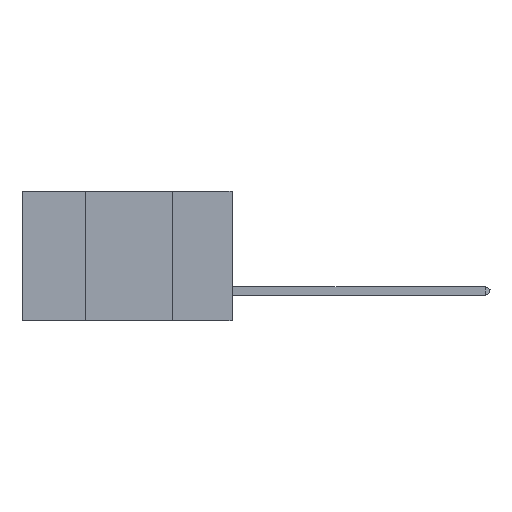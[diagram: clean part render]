
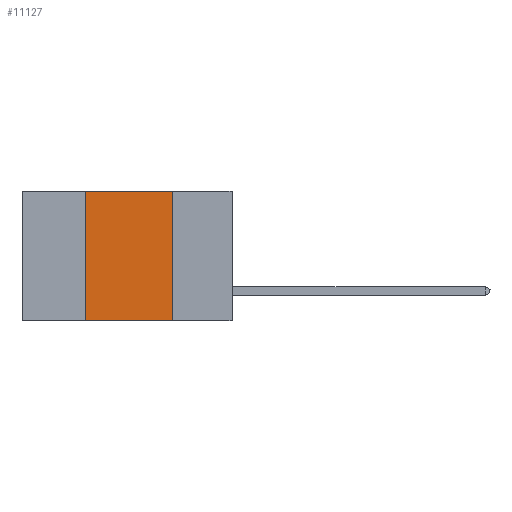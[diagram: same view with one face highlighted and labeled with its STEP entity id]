
A CAD part, left-side view. The second image highlights one B-rep face of the part: STEP entity #11127.
In plain terms, the highlighted planar face has unit normal (-1, 0, 0).
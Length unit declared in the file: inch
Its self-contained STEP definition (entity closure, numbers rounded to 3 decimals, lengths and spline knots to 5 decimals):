
#441 = ORIENTED_EDGE ( 'NONE', *, *, #6847, .F. ) ;
#1531 = CARTESIAN_POINT ( 'NONE',  ( 0., 0.42, -0.37 ) ) ;
#1762 = VERTEX_POINT ( 'NONE', #1531 ) ;
#2205 = LINE ( 'NONE', #15327, #3920 ) ;
#2285 = EDGE_CURVE ( 'NONE', #1762, #3247, #2205, .T. ) ;
#2792 = PLANE ( 'NONE',  #5983 ) ;
#3013 = CARTESIAN_POINT ( 'NONE',  ( 0., 0.6, 0. ) ) ;
#3247 = VERTEX_POINT ( 'NONE', #8377 ) ;
#3689 = LINE ( 'NONE', #3013, #16698 ) ;
#3920 = VECTOR ( 'NONE', #15156, 39.37008 ) ;
#4222 = DIRECTION ( 'NONE',  ( 1., 0., 0. ) ) ;
#4903 = CARTESIAN_POINT ( 'NONE',  ( 0., 0.17, 0. ) ) ;
#5390 = VERTEX_POINT ( 'NONE', #16232 ) ;
#5679 = CARTESIAN_POINT ( 'NONE',  ( 0., 0.42, 0. ) ) ;
#5760 = EDGE_CURVE ( 'NONE', #1762, #11812, #14618, .T. ) ;
#5983 = AXIS2_PLACEMENT_3D ( 'NONE', #8307, #4222, #11189 ) ;
#6644 = ORIENTED_EDGE ( 'NONE', *, *, #14881, .F. ) ;
#6847 = EDGE_CURVE ( 'NONE', #5390, #3247, #12910, .T. ) ;
#7449 = VECTOR ( 'NONE', #11631, 39.37008 ) ;
#8307 = CARTESIAN_POINT ( 'NONE',  ( 0., 0.6, 0. ) ) ;
#8377 = CARTESIAN_POINT ( 'NONE',  ( 0., 0.17, -0.37 ) ) ;
#9623 = FACE_OUTER_BOUND ( 'NONE', #12135, .T. ) ;
#11127 = ADVANCED_FACE ( 'NONE', ( #9623 ), #2792, .F. ) ;
#11189 = DIRECTION ( 'NONE',  ( 0., 0., -1. ) ) ;
#11302 = ORIENTED_EDGE ( 'NONE', *, *, #2285, .T. ) ;
#11413 = DIRECTION ( 'NONE',  ( 0., -1., 0. ) ) ;
#11631 = DIRECTION ( 'NONE',  ( 0., 0., -1. ) ) ;
#11720 = ORIENTED_EDGE ( 'NONE', *, *, #5760, .F. ) ;
#11812 = VERTEX_POINT ( 'NONE', #5679 ) ;
#12135 = EDGE_LOOP ( 'NONE', ( #441, #6644, #11720, #11302 ) ) ;
#12910 = LINE ( 'NONE', #4903, #7449 ) ;
#14618 = LINE ( 'NONE', #14785, #15722 ) ;
#14785 = CARTESIAN_POINT ( 'NONE',  ( 0., 0.42, 0. ) ) ;
#14860 = DIRECTION ( 'NONE',  ( 0., 0., 1. ) ) ;
#14881 = EDGE_CURVE ( 'NONE', #11812, #5390, #3689, .T. ) ;
#15156 = DIRECTION ( 'NONE',  ( 0., -1., 0. ) ) ;
#15327 = CARTESIAN_POINT ( 'NONE',  ( 0., 0.6, -0.37 ) ) ;
#15722 = VECTOR ( 'NONE', #14860, 39.37008 ) ;
#16232 = CARTESIAN_POINT ( 'NONE',  ( 0., 0.17, 0. ) ) ;
#16698 = VECTOR ( 'NONE', #11413, 39.37008 ) ;
